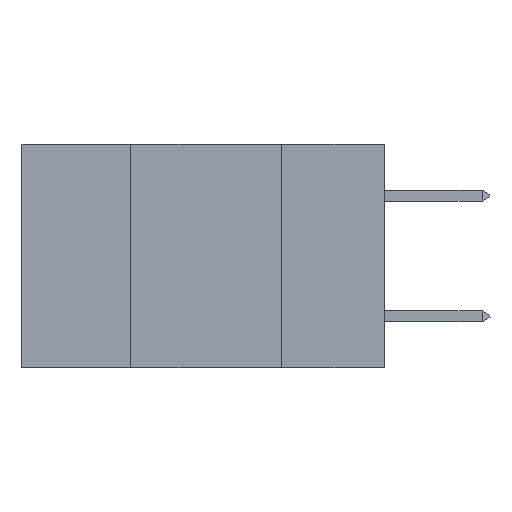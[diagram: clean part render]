
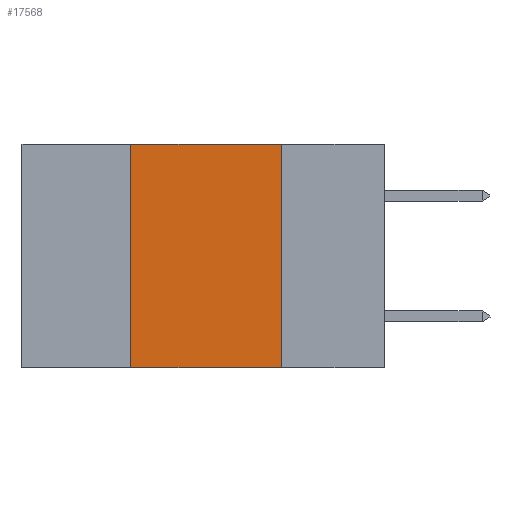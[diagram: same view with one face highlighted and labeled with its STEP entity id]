
A CAD part, left-side view. The second image highlights one B-rep face of the part: STEP entity #17568.
In plain terms, the highlighted planar face has unit normal (-1, 0, 0).
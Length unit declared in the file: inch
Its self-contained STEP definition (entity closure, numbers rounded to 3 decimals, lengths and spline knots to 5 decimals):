
#786 = VERTEX_POINT ( 'NONE', #12013 ) ;
#2411 = CARTESIAN_POINT ( 'NONE',  ( 0., 0.6, 0. ) ) ;
#2603 = AXIS2_PLACEMENT_3D ( 'NONE', #10452, #5132, #17572 ) ;
#3312 = CARTESIAN_POINT ( 'NONE',  ( 0., 0.17, 0. ) ) ;
#4333 = LINE ( 'NONE', #2411, #22632 ) ;
#4392 = VERTEX_POINT ( 'NONE', #9334 ) ;
#5132 = DIRECTION ( 'NONE',  ( 1., 0., 0. ) ) ;
#5327 = CARTESIAN_POINT ( 'NONE',  ( 0., 0.17, -0.37 ) ) ;
#6376 = EDGE_LOOP ( 'NONE', ( #11450, #14094, #14160, #14413 ) ) ;
#6556 = DIRECTION ( 'NONE',  ( 0., 0., -1. ) ) ;
#6883 = VERTEX_POINT ( 'NONE', #3312 ) ;
#6925 = VERTEX_POINT ( 'NONE', #5327 ) ;
#9334 = CARTESIAN_POINT ( 'NONE',  ( 0., 0.42, -0.37 ) ) ;
#9888 = CARTESIAN_POINT ( 'NONE',  ( 0., 0.6, -0.37 ) ) ;
#10439 = VECTOR ( 'NONE', #6556, 39.37008 ) ;
#10452 = CARTESIAN_POINT ( 'NONE',  ( 0., 0.6, 0. ) ) ;
#10850 = EDGE_CURVE ( 'NONE', #4392, #786, #12779, .T. ) ;
#11249 = CARTESIAN_POINT ( 'NONE',  ( 0., 0.42, 0. ) ) ;
#11450 = ORIENTED_EDGE ( 'NONE', *, *, #14461, .F. ) ;
#11636 = FACE_OUTER_BOUND ( 'NONE', #6376, .T. ) ;
#12013 = CARTESIAN_POINT ( 'NONE',  ( 0., 0.42, 0. ) ) ;
#12315 = EDGE_CURVE ( 'NONE', #786, #6883, #4333, .T. ) ;
#12779 = LINE ( 'NONE', #11249, #21590 ) ;
#13000 = DIRECTION ( 'NONE',  ( 0., 0., 1. ) ) ;
#13186 = DIRECTION ( 'NONE',  ( 0., -1., 0. ) ) ;
#13937 = VECTOR ( 'NONE', #15265, 39.37008 ) ;
#14094 = ORIENTED_EDGE ( 'NONE', *, *, #12315, .F. ) ;
#14160 = ORIENTED_EDGE ( 'NONE', *, *, #10850, .F. ) ;
#14413 = ORIENTED_EDGE ( 'NONE', *, *, #16180, .T. ) ;
#14461 = EDGE_CURVE ( 'NONE', #6883, #6925, #15182, .T. ) ;
#14513 = LINE ( 'NONE', #9888, #13937 ) ;
#15182 = LINE ( 'NONE', #18899, #10439 ) ;
#15265 = DIRECTION ( 'NONE',  ( 0., -1., 0. ) ) ;
#15819 = PLANE ( 'NONE',  #2603 ) ;
#16180 = EDGE_CURVE ( 'NONE', #4392, #6925, #14513, .T. ) ;
#17568 = ADVANCED_FACE ( 'NONE', ( #11636 ), #15819, .F. ) ;
#17572 = DIRECTION ( 'NONE',  ( 0., 0., -1. ) ) ;
#18899 = CARTESIAN_POINT ( 'NONE',  ( 0., 0.17, 0. ) ) ;
#21590 = VECTOR ( 'NONE', #13000, 39.37008 ) ;
#22632 = VECTOR ( 'NONE', #13186, 39.37008 ) ;
